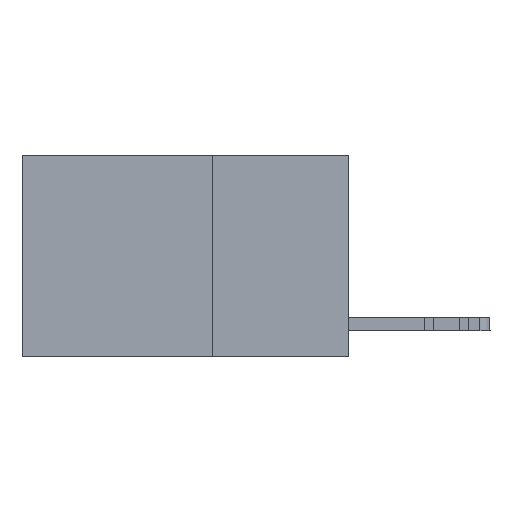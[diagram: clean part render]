
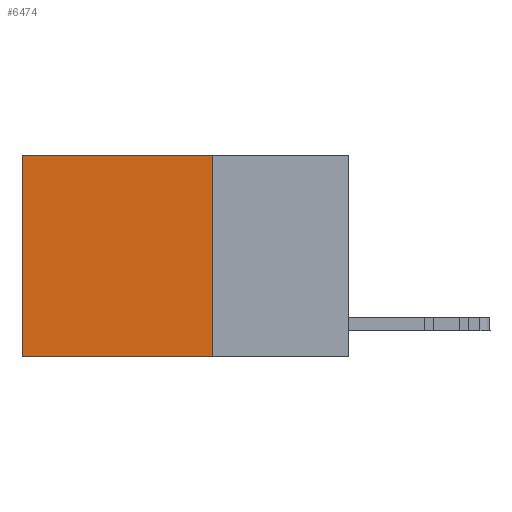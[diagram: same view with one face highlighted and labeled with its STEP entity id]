
A CAD part, left-side view. The second image highlights one B-rep face of the part: STEP entity #6474.
In plain terms, the highlighted planar face has unit normal (-1, 0, 0).
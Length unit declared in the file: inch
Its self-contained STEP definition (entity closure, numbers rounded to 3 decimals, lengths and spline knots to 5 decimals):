
#22 = ORIENTED_EDGE ( 'NONE', *, *, #18428, .F. ) ;
#100 = CARTESIAN_POINT ( 'NONE',  ( 0.2625, 0.25, 0. ) ) ;
#839 = EDGE_CURVE ( 'NONE', #3584, #30680, #23031, .T. ) ;
#873 = LINE ( 'NONE', #1180, #7222 ) ;
#1180 = CARTESIAN_POINT ( 'NONE',  ( 0.2625, 0.25, -0.37 ) ) ;
#1467 = CARTESIAN_POINT ( 'NONE',  ( 0.2625, 0.6, 0. ) ) ;
#1672 = CARTESIAN_POINT ( 'NONE',  ( 0.2625, 0.25, -0.37 ) ) ;
#2468 = DIRECTION ( 'NONE',  ( 0., 0., -1. ) ) ;
#2835 = ORIENTED_EDGE ( 'NONE', *, *, #839, .T. ) ;
#3584 = VERTEX_POINT ( 'NONE', #19857 ) ;
#4086 = DIRECTION ( 'NONE',  ( 1., 0., 0. ) ) ;
#6474 = ADVANCED_FACE ( 'NONE', ( #6893 ), #9245, .F. ) ;
#6893 = FACE_OUTER_BOUND ( 'NONE', #14164, .T. ) ;
#7073 = EDGE_CURVE ( 'NONE', #29977, #30680, #873, .T. ) ;
#7222 = VECTOR ( 'NONE', #22750, 39.37008 ) ;
#8082 = EDGE_CURVE ( 'NONE', #27170, #3584, #18523, .T. ) ;
#8612 = DIRECTION ( 'NONE',  ( 0., 1., 0. ) ) ;
#9245 = PLANE ( 'NONE',  #13197 ) ;
#13197 = AXIS2_PLACEMENT_3D ( 'NONE', #25628, #4086, #26080 ) ;
#13779 = VECTOR ( 'NONE', #16240, 39.37008 ) ;
#14164 = EDGE_LOOP ( 'NONE', ( #2835, #15880, #22, #17857 ) ) ;
#15615 = CARTESIAN_POINT ( 'NONE',  ( 0.2625, 0.6, -0.37 ) ) ;
#15858 = CARTESIAN_POINT ( 'NONE',  ( 0.2625, 0.25, 0. ) ) ;
#15880 = ORIENTED_EDGE ( 'NONE', *, *, #7073, .F. ) ;
#16240 = DIRECTION ( 'NONE',  ( 0., 0., -1. ) ) ;
#16533 = VECTOR ( 'NONE', #8612, 39.37008 ) ;
#17857 = ORIENTED_EDGE ( 'NONE', *, *, #8082, .T. ) ;
#18428 = EDGE_CURVE ( 'NONE', #27170, #29977, #27159, .T. ) ;
#18523 = LINE ( 'NONE', #15858, #16533 ) ;
#18540 = VECTOR ( 'NONE', #2468, 39.37008 ) ;
#19857 = CARTESIAN_POINT ( 'NONE',  ( 0.2625, 0.6, 0. ) ) ;
#22750 = DIRECTION ( 'NONE',  ( 0., 1., 0. ) ) ;
#23031 = LINE ( 'NONE', #1467, #13779 ) ;
#24410 = CARTESIAN_POINT ( 'NONE',  ( 0.2625, 0.25, 0. ) ) ;
#25628 = CARTESIAN_POINT ( 'NONE',  ( 0.2625, 0.25, 0. ) ) ;
#26080 = DIRECTION ( 'NONE',  ( 0., 0., -1. ) ) ;
#27159 = LINE ( 'NONE', #100, #18540 ) ;
#27170 = VERTEX_POINT ( 'NONE', #24410 ) ;
#29977 = VERTEX_POINT ( 'NONE', #1672 ) ;
#30680 = VERTEX_POINT ( 'NONE', #15615 ) ;
